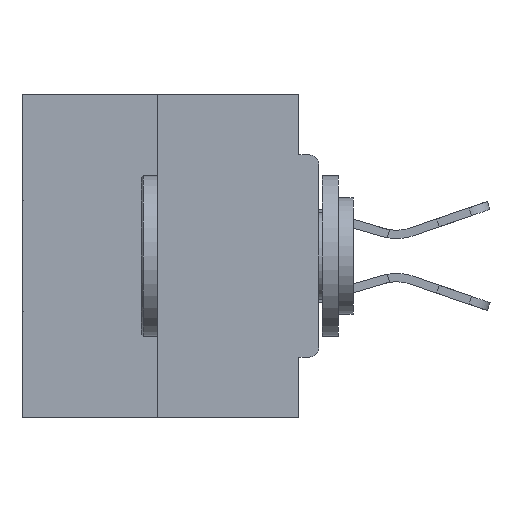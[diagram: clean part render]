
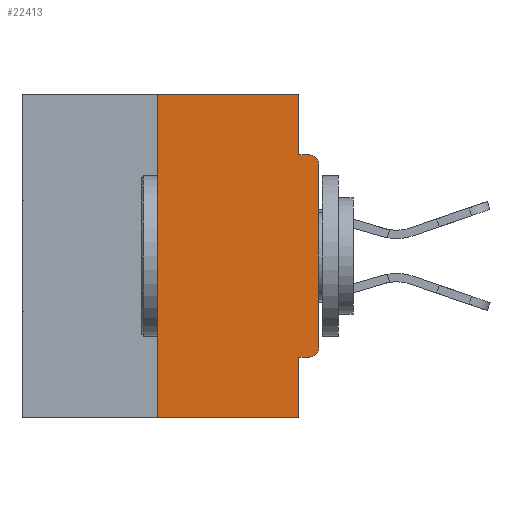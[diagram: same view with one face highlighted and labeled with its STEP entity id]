
A CAD part, left-side view. The second image highlights one B-rep face of the part: STEP entity #22413.
In plain terms, the highlighted planar face has unit normal (-1, 0, 0).
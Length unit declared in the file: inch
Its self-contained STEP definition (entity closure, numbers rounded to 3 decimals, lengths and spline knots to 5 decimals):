
#781 = CARTESIAN_POINT ( 'NONE',  ( 0., 0.031, 0. ) ) ;
#1086 = LINE ( 'NONE', #16898, #12049 ) ;
#1572 = ORIENTED_EDGE ( 'NONE', *, *, #25124, .T. ) ;
#3042 = EDGE_CURVE ( 'NONE', #13453, #32329, #21491, .T. ) ;
#3264 = PLANE ( 'NONE',  #38248 ) ;
#3840 = EDGE_CURVE ( 'NONE', #13453, #11415, #30472, .T. ) ;
#4131 = VERTEX_POINT ( 'NONE', #5850 ) ;
#5002 = DIRECTION ( 'NONE',  ( 0., 0., -1. ) ) ;
#5242 = DIRECTION ( 'NONE',  ( -1., 0., 0. ) ) ;
#5508 = DIRECTION ( 'NONE',  ( 0., 0., -1. ) ) ;
#5850 = CARTESIAN_POINT ( 'NONE',  ( 0., 0.031, -0.0935 ) ) ;
#5851 = CARTESIAN_POINT ( 'NONE',  ( 0., 0.031, -0.4065 ) ) ;
#6643 = VECTOR ( 'NONE', #34545, 39.37008 ) ;
#6712 = ORIENTED_EDGE ( 'NONE', *, *, #23359, .T. ) ;
#6919 = LINE ( 'NONE', #12038, #38863 ) ;
#7250 = CARTESIAN_POINT ( 'NONE',  ( 0., 0., 0. ) ) ;
#8753 = VERTEX_POINT ( 'NONE', #5851 ) ;
#8826 = VERTEX_POINT ( 'NONE', #33172 ) ;
#10966 = CARTESIAN_POINT ( 'NONE',  ( 0., 0.015, -0.1085 ) ) ;
#11415 = VERTEX_POINT ( 'NONE', #32485 ) ;
#11877 = DIRECTION ( 'NONE',  ( 0., 0., -1. ) ) ;
#11889 = VECTOR ( 'NONE', #29844, 39.37008 ) ;
#12038 = CARTESIAN_POINT ( 'NONE',  ( 0., 0.031, 0. ) ) ;
#12049 = VECTOR ( 'NONE', #14077, 39.37008 ) ;
#12936 = ORIENTED_EDGE ( 'NONE', *, *, #24604, .F. ) ;
#13453 = VERTEX_POINT ( 'NONE', #25871 ) ;
#14077 = DIRECTION ( 'NONE',  ( 0., -1., 0. ) ) ;
#14502 = DIRECTION ( 'NONE',  ( 0., -1., 0. ) ) ;
#14566 = CARTESIAN_POINT ( 'NONE',  ( 0., 0.031, -0.5 ) ) ;
#14816 = DIRECTION ( 'NONE',  ( 1., 0., 0. ) ) ;
#16720 = EDGE_CURVE ( 'NONE', #11415, #17893, #1086, .T. ) ;
#16832 = DIRECTION ( 'NONE',  ( 0., 0., -1. ) ) ;
#16898 = CARTESIAN_POINT ( 'NONE',  ( 0., 0.46, 0. ) ) ;
#16970 = ORIENTED_EDGE ( 'NONE', *, *, #22251, .T. ) ;
#17893 = VERTEX_POINT ( 'NONE', #781 ) ;
#18755 = VECTOR ( 'NONE', #31122, 39.37008 ) ;
#19084 = AXIS2_PLACEMENT_3D ( 'NONE', #23457, #5242, #5508 ) ;
#20731 = CIRCLE ( 'NONE', #39488, 0.015 ) ;
#21491 = LINE ( 'NONE', #36155, #35829 ) ;
#21829 = ORIENTED_EDGE ( 'NONE', *, *, #31457, .F. ) ;
#22251 = EDGE_CURVE ( 'NONE', #37537, #8826, #30369, .T. ) ;
#22413 = ADVANCED_FACE ( 'NONE', ( #33245 ), #3264, .F. ) ;
#23047 = VECTOR ( 'NONE', #34665, 39.37008 ) ;
#23359 = EDGE_CURVE ( 'NONE', #29862, #26286, #20731, .T. ) ;
#23457 = CARTESIAN_POINT ( 'NONE',  ( 0., 0.015, -0.3915 ) ) ;
#23614 = ORIENTED_EDGE ( 'NONE', *, *, #36179, .F. ) ;
#23861 = ORIENTED_EDGE ( 'NONE', *, *, #3840, .F. ) ;
#24083 = CARTESIAN_POINT ( 'NONE',  ( 0., 0., -0.0935 ) ) ;
#24498 = ORIENTED_EDGE ( 'NONE', *, *, #31543, .F. ) ;
#24604 = EDGE_CURVE ( 'NONE', #37537, #8753, #37391, .T. ) ;
#25064 = CARTESIAN_POINT ( 'NONE',  ( 0., 0.015, -0.4065 ) ) ;
#25124 = EDGE_CURVE ( 'NONE', #8826, #29862, #30684, .T. ) ;
#25521 = VECTOR ( 'NONE', #5002, 39.37008 ) ;
#25871 = CARTESIAN_POINT ( 'NONE',  ( 0., 0.25, -0.5 ) ) ;
#26286 = VERTEX_POINT ( 'NONE', #29430 ) ;
#26383 = EDGE_LOOP ( 'NONE', ( #33216, #23861, #28547, #21829, #12936, #16970, #1572, #6712, #23614, #24498 ) ) ;
#26487 = LINE ( 'NONE', #14566, #25521 ) ;
#27100 = CARTESIAN_POINT ( 'NONE',  ( 0., 0.46, 0. ) ) ;
#28547 = ORIENTED_EDGE ( 'NONE', *, *, #3042, .T. ) ;
#29430 = CARTESIAN_POINT ( 'NONE',  ( 0., 0.015, -0.0935 ) ) ;
#29844 = DIRECTION ( 'NONE',  ( 0., -1., 0. ) ) ;
#29862 = VERTEX_POINT ( 'NONE', #31526 ) ;
#30369 = CIRCLE ( 'NONE', #19084, 0.015 ) ;
#30472 = LINE ( 'NONE', #37340, #6643 ) ;
#30684 = LINE ( 'NONE', #7250, #18755 ) ;
#31122 = DIRECTION ( 'NONE',  ( 0., 0., 1. ) ) ;
#31297 = CARTESIAN_POINT ( 'NONE',  ( 0., 0.031, -0.5 ) ) ;
#31457 = EDGE_CURVE ( 'NONE', #8753, #32329, #26487, .T. ) ;
#31526 = CARTESIAN_POINT ( 'NONE',  ( 0., 0., -0.1085 ) ) ;
#31543 = EDGE_CURVE ( 'NONE', #17893, #4131, #6919, .T. ) ;
#32329 = VERTEX_POINT ( 'NONE', #31297 ) ;
#32485 = CARTESIAN_POINT ( 'NONE',  ( 0., 0.25, 0. ) ) ;
#33172 = CARTESIAN_POINT ( 'NONE',  ( 0., 0., -0.3915 ) ) ;
#33216 = ORIENTED_EDGE ( 'NONE', *, *, #16720, .F. ) ;
#33245 = FACE_OUTER_BOUND ( 'NONE', #26383, .T. ) ;
#33382 = DIRECTION ( 'NONE',  ( 0., 0., -1. ) ) ;
#34545 = DIRECTION ( 'NONE',  ( 0., 0., 1. ) ) ;
#34665 = DIRECTION ( 'NONE',  ( 0., 1., 0. ) ) ;
#34795 = CARTESIAN_POINT ( 'NONE',  ( 0., 0., -0.4065 ) ) ;
#35829 = VECTOR ( 'NONE', #14502, 39.37008 ) ;
#36155 = CARTESIAN_POINT ( 'NONE',  ( 0., 0.46, -0.5 ) ) ;
#36179 = EDGE_CURVE ( 'NONE', #4131, #26286, #38633, .T. ) ;
#37340 = CARTESIAN_POINT ( 'NONE',  ( 0., 0.25, 0. ) ) ;
#37391 = LINE ( 'NONE', #34795, #23047 ) ;
#37537 = VERTEX_POINT ( 'NONE', #25064 ) ;
#37905 = DIRECTION ( 'NONE',  ( -1., 0., 0. ) ) ;
#38248 = AXIS2_PLACEMENT_3D ( 'NONE', #27100, #14816, #11877 ) ;
#38633 = LINE ( 'NONE', #24083, #11889 ) ;
#38863 = VECTOR ( 'NONE', #33382, 39.37008 ) ;
#39488 = AXIS2_PLACEMENT_3D ( 'NONE', #10966, #37905, #16832 ) ;
